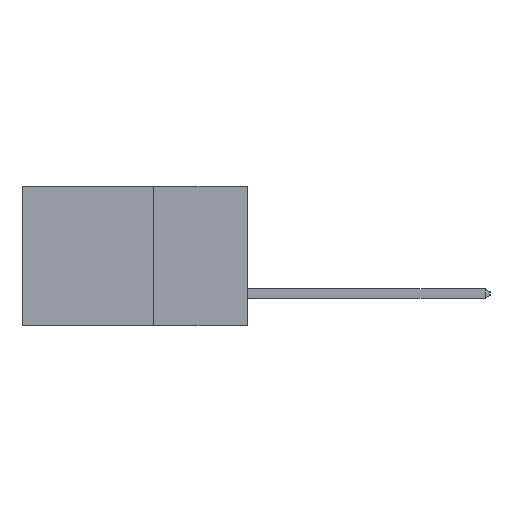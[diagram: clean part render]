
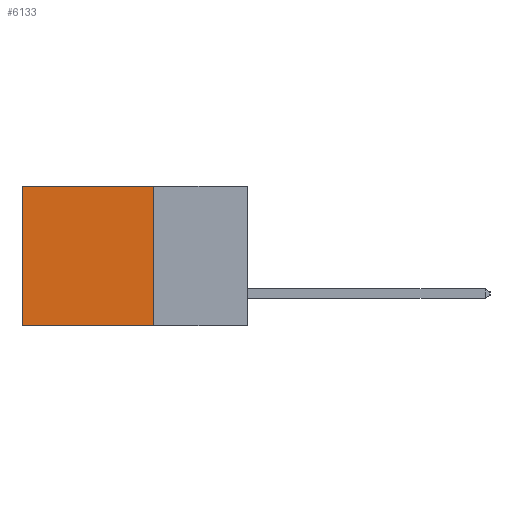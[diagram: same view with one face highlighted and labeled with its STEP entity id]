
A CAD part, left-side view. The second image highlights one B-rep face of the part: STEP entity #6133.
In plain terms, the highlighted planar face has unit normal (-1, 0, 0).
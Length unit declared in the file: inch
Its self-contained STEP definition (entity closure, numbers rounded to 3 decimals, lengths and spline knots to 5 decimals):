
#93 = CARTESIAN_POINT ( 'NONE',  ( 0.298, 0.25, -0.37 ) ) ;
#404 = EDGE_CURVE ( 'NONE', #4497, #464, #7946, .T. ) ;
#464 = VERTEX_POINT ( 'NONE', #8184 ) ;
#1096 = CARTESIAN_POINT ( 'NONE',  ( 0.298, 0.25, -0.37 ) ) ;
#1361 = VERTEX_POINT ( 'NONE', #93 ) ;
#1464 = VECTOR ( 'NONE', #9819, 39.37008 ) ;
#1767 = EDGE_LOOP ( 'NONE', ( #6255, #6302, #6324, #6485 ) ) ;
#1826 = EDGE_CURVE ( 'NONE', #4211, #4497, #7465, .T. ) ;
#2235 = VECTOR ( 'NONE', #8972, 39.37008 ) ;
#2278 = PLANE ( 'NONE',  #8759 ) ;
#3154 = CARTESIAN_POINT ( 'NONE',  ( 0.298, 0.6, 0. ) ) ;
#3682 = CARTESIAN_POINT ( 'NONE',  ( 0.298, 0.25, 0. ) ) ;
#4211 = VERTEX_POINT ( 'NONE', #3682 ) ;
#4470 = DIRECTION ( 'NONE',  ( 1., 0., 0. ) ) ;
#4497 = VERTEX_POINT ( 'NONE', #3154 ) ;
#5070 = LINE ( 'NONE', #1096, #2235 ) ;
#5314 = EDGE_CURVE ( 'NONE', #1361, #464, #5070, .T. ) ;
#5513 = VECTOR ( 'NONE', #10696, 39.37008 ) ;
#5602 = VECTOR ( 'NONE', #10346, 39.37008 ) ;
#5649 = FACE_OUTER_BOUND ( 'NONE', #1767, .T. ) ;
#6133 = ADVANCED_FACE ( 'NONE', ( #5649 ), #2278, .F. ) ;
#6255 = ORIENTED_EDGE ( 'NONE', *, *, #404, .T. ) ;
#6302 = ORIENTED_EDGE ( 'NONE', *, *, #5314, .F. ) ;
#6324 = ORIENTED_EDGE ( 'NONE', *, *, #11282, .F. ) ;
#6485 = ORIENTED_EDGE ( 'NONE', *, *, #1826, .T. ) ;
#6614 = CARTESIAN_POINT ( 'NONE',  ( 0.298, 0.6, 0. ) ) ;
#7227 = CARTESIAN_POINT ( 'NONE',  ( 0.298, 0.25, 0. ) ) ;
#7465 = LINE ( 'NONE', #11554, #5602 ) ;
#7946 = LINE ( 'NONE', #6614, #5513 ) ;
#8184 = CARTESIAN_POINT ( 'NONE',  ( 0.298, 0.6, -0.37 ) ) ;
#8759 = AXIS2_PLACEMENT_3D ( 'NONE', #9033, #4470, #10700 ) ;
#8972 = DIRECTION ( 'NONE',  ( 0., 1., 0. ) ) ;
#9033 = CARTESIAN_POINT ( 'NONE',  ( 0.298, 0.25, 0. ) ) ;
#9239 = LINE ( 'NONE', #7227, #1464 ) ;
#9819 = DIRECTION ( 'NONE',  ( 0., 0., -1. ) ) ;
#10346 = DIRECTION ( 'NONE',  ( 0., 1., 0. ) ) ;
#10696 = DIRECTION ( 'NONE',  ( 0., 0., -1. ) ) ;
#10700 = DIRECTION ( 'NONE',  ( 0., 0., -1. ) ) ;
#11282 = EDGE_CURVE ( 'NONE', #4211, #1361, #9239, .T. ) ;
#11554 = CARTESIAN_POINT ( 'NONE',  ( 0.298, 0.25, 0. ) ) ;
